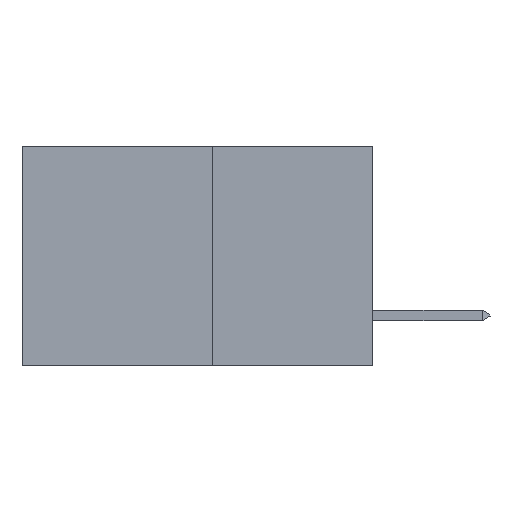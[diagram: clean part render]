
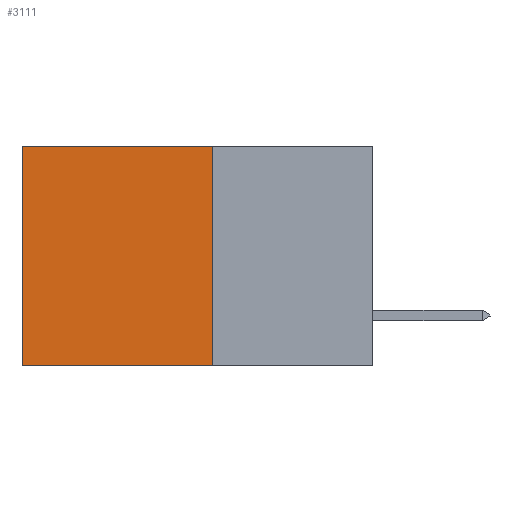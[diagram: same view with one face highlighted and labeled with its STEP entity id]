
A CAD part, left-side view. The second image highlights one B-rep face of the part: STEP entity #3111.
In plain terms, the highlighted planar face has unit normal (-1, 0, 0).
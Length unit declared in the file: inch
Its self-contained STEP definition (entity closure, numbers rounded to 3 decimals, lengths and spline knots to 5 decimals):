
#42 = CARTESIAN_POINT ( 'NONE',  ( 0.277, 0.59, -0.37 ) ) ;
#73 = VERTEX_POINT ( 'NONE', #7744 ) ;
#441 = CARTESIAN_POINT ( 'NONE',  ( 0.277, 0.59, -0.37 ) ) ;
#699 = DIRECTION ( 'NONE',  ( 0., 1., 0. ) ) ;
#718 = CARTESIAN_POINT ( 'NONE',  ( 0.277, 0.27, -0.37 ) ) ;
#2112 = DIRECTION ( 'NONE',  ( 1., 0., 0. ) ) ;
#2628 = LINE ( 'NONE', #10137, #14359 ) ;
#3024 = EDGE_CURVE ( 'NONE', #6735, #3321, #2628, .T. ) ;
#3111 = ADVANCED_FACE ( 'NONE', ( #13681 ), #9145, .F. ) ;
#3321 = VERTEX_POINT ( 'NONE', #10528 ) ;
#3441 = LINE ( 'NONE', #6205, #12210 ) ;
#4397 = DIRECTION ( 'NONE',  ( 0., 0., -1. ) ) ;
#4693 = EDGE_CURVE ( 'NONE', #6735, #73, #11431, .T. ) ;
#4957 = VERTEX_POINT ( 'NONE', #42 ) ;
#6205 = CARTESIAN_POINT ( 'NONE',  ( 0.277, 0.27, -0.37 ) ) ;
#6735 = VERTEX_POINT ( 'NONE', #10950 ) ;
#6897 = EDGE_CURVE ( 'NONE', #73, #4957, #12959, .T. ) ;
#7744 = CARTESIAN_POINT ( 'NONE',  ( 0.277, 0.59, 0. ) ) ;
#8149 = ORIENTED_EDGE ( 'NONE', *, *, #3024, .F. ) ;
#9007 = AXIS2_PLACEMENT_3D ( 'NONE', #718, #2112, #10280 ) ;
#9145 = PLANE ( 'NONE',  #9007 ) ;
#10059 = DIRECTION ( 'NONE',  ( 0., 0., -1. ) ) ;
#10137 = CARTESIAN_POINT ( 'NONE',  ( 0.277, 0.27, -0.37 ) ) ;
#10280 = DIRECTION ( 'NONE',  ( 0., 0., -1. ) ) ;
#10528 = CARTESIAN_POINT ( 'NONE',  ( 0.277, 0.27, -0.37 ) ) ;
#10701 = DIRECTION ( 'NONE',  ( 0., 1., 0. ) ) ;
#10950 = CARTESIAN_POINT ( 'NONE',  ( 0.277, 0.27, 0. ) ) ;
#11343 = CARTESIAN_POINT ( 'NONE',  ( 0.277, 0.27, 0. ) ) ;
#11431 = LINE ( 'NONE', #11343, #13990 ) ;
#12083 = EDGE_CURVE ( 'NONE', #3321, #4957, #3441, .T. ) ;
#12210 = VECTOR ( 'NONE', #10701, 39.37008 ) ;
#12617 = VECTOR ( 'NONE', #10059, 39.37008 ) ;
#12959 = LINE ( 'NONE', #441, #12617 ) ;
#13681 = FACE_OUTER_BOUND ( 'NONE', #13868, .T. ) ;
#13868 = EDGE_LOOP ( 'NONE', ( #13881, #14852, #8149, #14599 ) ) ;
#13881 = ORIENTED_EDGE ( 'NONE', *, *, #6897, .T. ) ;
#13990 = VECTOR ( 'NONE', #699, 39.37008 ) ;
#14359 = VECTOR ( 'NONE', #4397, 39.37008 ) ;
#14599 = ORIENTED_EDGE ( 'NONE', *, *, #4693, .T. ) ;
#14852 = ORIENTED_EDGE ( 'NONE', *, *, #12083, .F. ) ;
